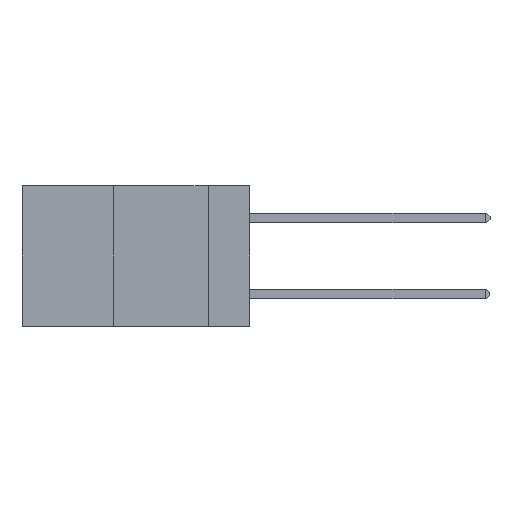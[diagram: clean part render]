
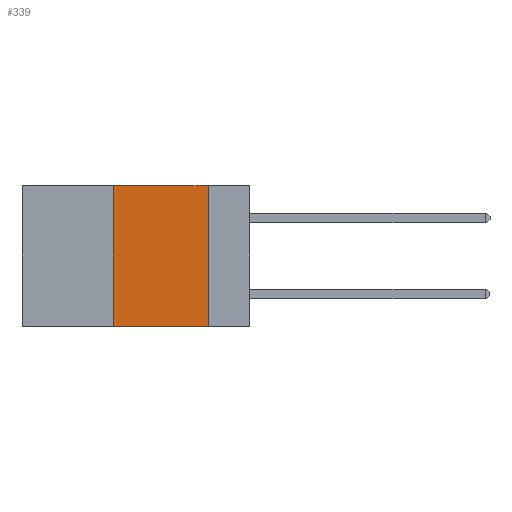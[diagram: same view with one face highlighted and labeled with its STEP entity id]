
A CAD part, left-side view. The second image highlights one B-rep face of the part: STEP entity #339.
In plain terms, the highlighted planar face has unit normal (-1, 0, 0).
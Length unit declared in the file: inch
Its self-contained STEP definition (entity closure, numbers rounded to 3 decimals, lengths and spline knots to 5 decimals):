
#9 = DIRECTION ( 'NONE',  ( 0., -1., 0. ) ) ;
#104 = ORIENTED_EDGE ( 'NONE', *, *, #5792, .T. ) ;
#274 = VECTOR ( 'NONE', #7788, 39.37008 ) ;
#339 = ADVANCED_FACE ( 'NONE', ( #836 ), #5412, .F. ) ;
#719 = CARTESIAN_POINT ( 'NONE',  ( 0., 0.6, -0.37 ) ) ;
#836 = FACE_OUTER_BOUND ( 'NONE', #6545, .T. ) ;
#858 = VERTEX_POINT ( 'NONE', #6542 ) ;
#983 = EDGE_CURVE ( 'NONE', #858, #8935, #4472, .T. ) ;
#1174 = LINE ( 'NONE', #7565, #6956 ) ;
#1398 = VERTEX_POINT ( 'NONE', #4519 ) ;
#1740 = ORIENTED_EDGE ( 'NONE', *, *, #983, .F. ) ;
#1932 = ORIENTED_EDGE ( 'NONE', *, *, #4879, .F. ) ;
#2182 = ORIENTED_EDGE ( 'NONE', *, *, #7432, .F. ) ;
#3550 = DIRECTION ( 'NONE',  ( 0., 0., -1. ) ) ;
#4327 = LINE ( 'NONE', #5042, #5936 ) ;
#4439 = VERTEX_POINT ( 'NONE', #4829 ) ;
#4461 = AXIS2_PLACEMENT_3D ( 'NONE', #7363, #6376, #7485 ) ;
#4472 = LINE ( 'NONE', #4729, #274 ) ;
#4519 = CARTESIAN_POINT ( 'NONE',  ( 0., 0.36, -0.37 ) ) ;
#4729 = CARTESIAN_POINT ( 'NONE',  ( 0., 0.6, 0. ) ) ;
#4802 = DIRECTION ( 'NONE',  ( 0., 0., 1. ) ) ;
#4829 = CARTESIAN_POINT ( 'NONE',  ( 0., 0.11, -0.37 ) ) ;
#4879 = EDGE_CURVE ( 'NONE', #1398, #858, #4327, .T. ) ;
#5042 = CARTESIAN_POINT ( 'NONE',  ( 0., 0.36, 0. ) ) ;
#5285 = VECTOR ( 'NONE', #9, 39.37008 ) ;
#5412 = PLANE ( 'NONE',  #4461 ) ;
#5792 = EDGE_CURVE ( 'NONE', #1398, #4439, #7087, .T. ) ;
#5936 = VECTOR ( 'NONE', #4802, 39.37008 ) ;
#6376 = DIRECTION ( 'NONE',  ( 1., 0., 0. ) ) ;
#6542 = CARTESIAN_POINT ( 'NONE',  ( 0., 0.36, 0. ) ) ;
#6545 = EDGE_LOOP ( 'NONE', ( #2182, #1740, #1932, #104 ) ) ;
#6956 = VECTOR ( 'NONE', #3550, 39.37008 ) ;
#7087 = LINE ( 'NONE', #719, #5285 ) ;
#7363 = CARTESIAN_POINT ( 'NONE',  ( 0., 0.6, 0. ) ) ;
#7432 = EDGE_CURVE ( 'NONE', #8935, #4439, #1174, .T. ) ;
#7485 = DIRECTION ( 'NONE',  ( 0., 0., -1. ) ) ;
#7565 = CARTESIAN_POINT ( 'NONE',  ( 0., 0.11, 0. ) ) ;
#7788 = DIRECTION ( 'NONE',  ( 0., -1., 0. ) ) ;
#8035 = CARTESIAN_POINT ( 'NONE',  ( 0., 0.11, 0. ) ) ;
#8935 = VERTEX_POINT ( 'NONE', #8035 ) ;
